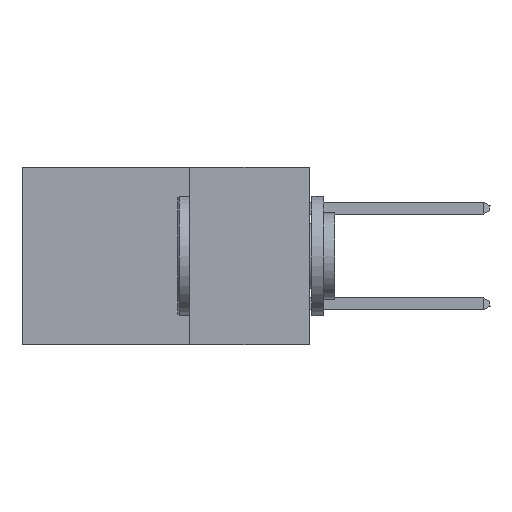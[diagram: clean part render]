
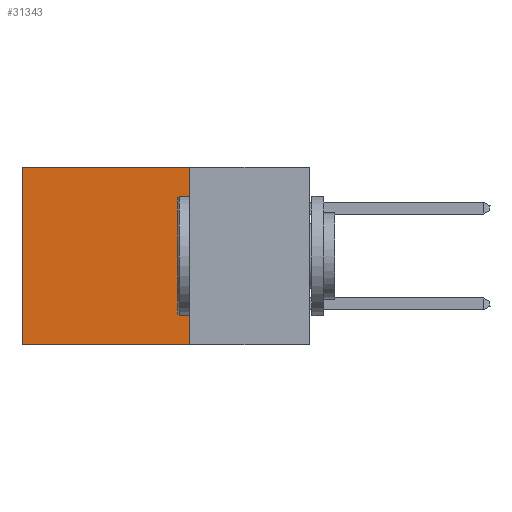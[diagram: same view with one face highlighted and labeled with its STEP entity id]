
A CAD part, left-side view. The second image highlights one B-rep face of the part: STEP entity #31343.
In plain terms, the highlighted planar face has unit normal (-1, 0, 0).
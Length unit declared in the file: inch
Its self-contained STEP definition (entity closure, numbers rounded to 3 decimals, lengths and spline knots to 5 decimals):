
#87 = EDGE_CURVE ( 'NONE', #43861, #35013, #6626, .T. ) ;
#1462 = DIRECTION ( 'NONE',  ( 0., 0., -1. ) ) ;
#2396 = LINE ( 'NONE', #6621, #30723 ) ;
#5031 = VECTOR ( 'NONE', #42775, 39.37008 ) ;
#6451 = LINE ( 'NONE', #28968, #43136 ) ;
#6621 = CARTESIAN_POINT ( 'NONE',  ( 0.2875, 0.6, 0. ) ) ;
#6626 = LINE ( 'NONE', #39084, #5031 ) ;
#6654 = EDGE_CURVE ( 'NONE', #38179, #40918, #2396, .T. ) ;
#10038 = EDGE_CURVE ( 'NONE', #43861, #38179, #44295, .T. ) ;
#11535 = DIRECTION ( 'NONE',  ( 0., 0., -1. ) ) ;
#11878 = CARTESIAN_POINT ( 'NONE',  ( 0.2875, 0.6, 0. ) ) ;
#12613 = CARTESIAN_POINT ( 'NONE',  ( 0.2875, 0.25, 0. ) ) ;
#15872 = PLANE ( 'NONE',  #21475 ) ;
#16227 = ORIENTED_EDGE ( 'NONE', *, *, #23712, .F. ) ;
#20912 = FACE_OUTER_BOUND ( 'NONE', #29627, .T. ) ;
#21452 = DIRECTION ( 'NONE',  ( 0., 1., 0. ) ) ;
#21475 = AXIS2_PLACEMENT_3D ( 'NONE', #12613, #26434, #1462 ) ;
#23712 = EDGE_CURVE ( 'NONE', #35013, #40918, #6451, .T. ) ;
#26434 = DIRECTION ( 'NONE',  ( 1., 0., 0. ) ) ;
#28043 = CARTESIAN_POINT ( 'NONE',  ( 0.2875, 0.6, -0.37 ) ) ;
#28968 = CARTESIAN_POINT ( 'NONE',  ( 0.2875, 0.25, -0.37 ) ) ;
#29627 = EDGE_LOOP ( 'NONE', ( #43937, #16227, #36616, #41559 ) ) ;
#30307 = CARTESIAN_POINT ( 'NONE',  ( 0.2875, 0.25, 0. ) ) ;
#30723 = VECTOR ( 'NONE', #11535, 39.37008 ) ;
#31343 = ADVANCED_FACE ( 'NONE', ( #20912 ), #15872, .F. ) ;
#35013 = VERTEX_POINT ( 'NONE', #39969 ) ;
#36616 = ORIENTED_EDGE ( 'NONE', *, *, #87, .F. ) ;
#38179 = VERTEX_POINT ( 'NONE', #11878 ) ;
#38238 = VECTOR ( 'NONE', #38971, 39.37008 ) ;
#38971 = DIRECTION ( 'NONE',  ( 0., 1., 0. ) ) ;
#39084 = CARTESIAN_POINT ( 'NONE',  ( 0.2875, 0.25, 0. ) ) ;
#39969 = CARTESIAN_POINT ( 'NONE',  ( 0.2875, 0.25, -0.37 ) ) ;
#40918 = VERTEX_POINT ( 'NONE', #28043 ) ;
#41559 = ORIENTED_EDGE ( 'NONE', *, *, #10038, .T. ) ;
#42775 = DIRECTION ( 'NONE',  ( 0., 0., -1. ) ) ;
#43136 = VECTOR ( 'NONE', #21452, 39.37008 ) ;
#43219 = CARTESIAN_POINT ( 'NONE',  ( 0.2875, 0.25, 0. ) ) ;
#43861 = VERTEX_POINT ( 'NONE', #43219 ) ;
#43937 = ORIENTED_EDGE ( 'NONE', *, *, #6654, .T. ) ;
#44295 = LINE ( 'NONE', #30307, #38238 ) ;
